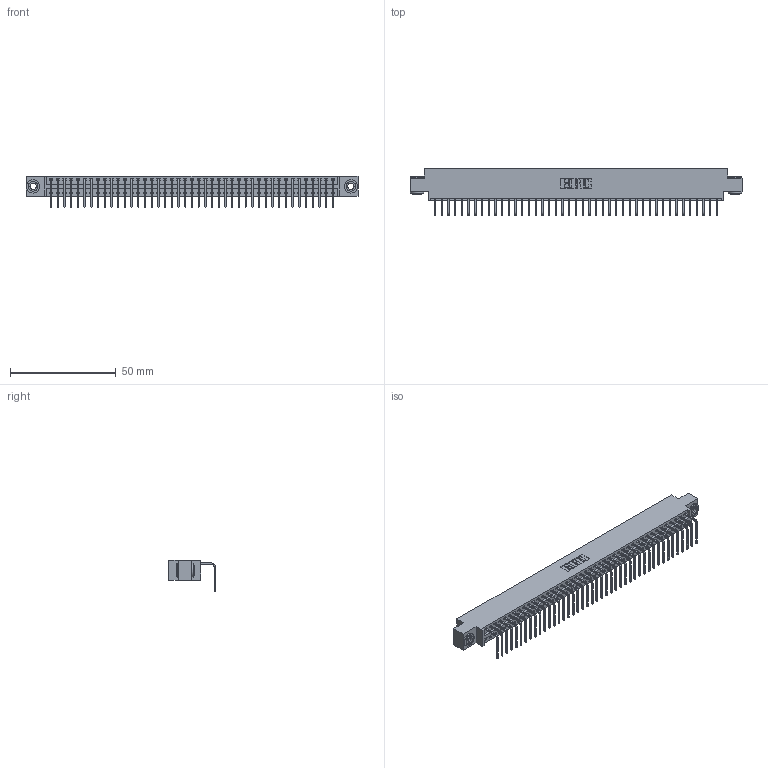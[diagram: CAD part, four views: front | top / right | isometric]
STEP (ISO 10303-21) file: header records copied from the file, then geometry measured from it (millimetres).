
FILE_DESCRIPTION (( 'STEP AP203' ), '1' );
FILE_NAME ('396-043-558-603.STEP', '2019-11-01T08:02:31', ( '' ), ( '' ), 'SwSTEP 2.0', 'SolidWorks 2016', '' );
FILE_SCHEMA (( 'CONFIG_CONTROL_DESIGN' ));
Length unit declared in the file: inch
Products named in the file (4): 345-292-001_558 Tail - 2; 345-250-002_345-250-002-102; 396-043-558-603; 346 Part_0.170 Offset - 0.156 Dia-TH
Assembly tree (46 placements, depth 2):
  396-043-558-603
    346 Part_0.170 Offset - 0.156 Dia-TH
    345-292-001_558 Tail - 2  x43
    345-250-002_345-250-002-102  x2
Bounding box: 157.1 x 22.16 x 14.73 mm (x, y, z)
Volume: 15052.8 mm3; surface area: 20059 mm2
Topology: 46 solids, 46 shells, 2744 faces, 8243 edges, 5434 vertices
Faces by surface type: plane 1896, cylinder 840, cone 8
Entity records: 27418 total; most frequent: CARTESIAN_POINT 4680, ORIENTED_EDGE 4650, DIRECTION 4157, EDGE_CURVE 2325, LINE 1997, VECTOR 1997, VERTEX_POINT 1546, AXIS2_PLACEMENT_3D 1080
